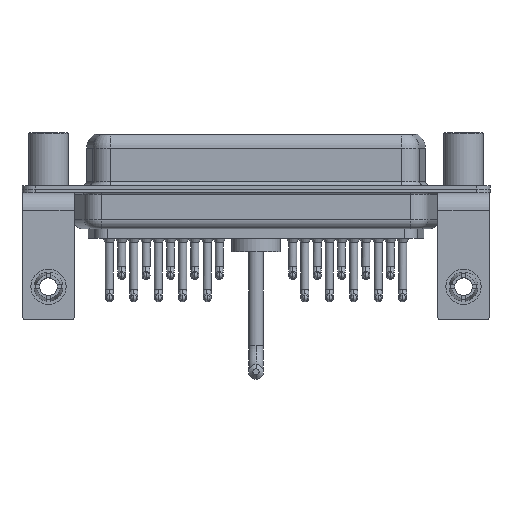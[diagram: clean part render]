
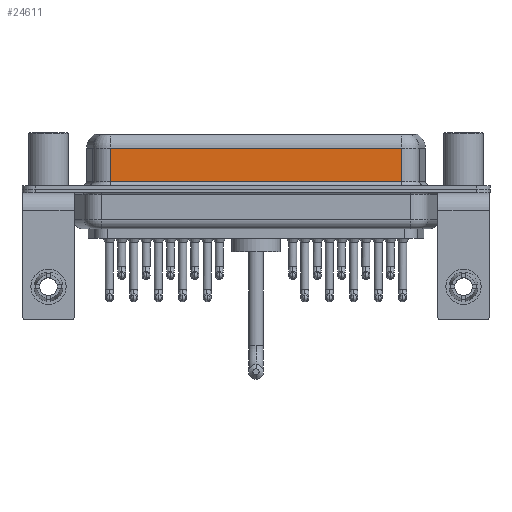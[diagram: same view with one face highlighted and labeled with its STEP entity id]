
A CAD part, front view. The second image highlights one B-rep face of the part: STEP entity #24611.
In plain terms, the highlighted planar face has unit normal (0, -1, 0).
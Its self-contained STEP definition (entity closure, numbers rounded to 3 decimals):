
#1301 = DIRECTION ( 'NONE',  ( 0., 0., 1. ) ) ;
#2319 = DIRECTION ( 'NONE',  ( 1., 0., 0. ) ) ;
#3087 = ORIENTED_EDGE ( 'NONE', *, *, #19730, .T. ) ;
#3514 = EDGE_CURVE ( 'NONE', #24640, #5284, #23763, .T. ) ;
#4156 = CARTESIAN_POINT ( 'NONE',  ( 40.037, -3.95, 4.65 ) ) ;
#4439 = ORIENTED_EDGE ( 'NONE', *, *, #3514, .T. ) ;
#4939 = LINE ( 'NONE', #9287, #15306 ) ;
#5242 = CARTESIAN_POINT ( 'NONE',  ( 7.013, -3.95, 4.65 ) ) ;
#5284 = VERTEX_POINT ( 'NONE', #23367 ) ;
#5513 = FACE_OUTER_BOUND ( 'NONE', #15312, .T. ) ;
#6496 = LINE ( 'NONE', #8418, #7118 ) ;
#7118 = VECTOR ( 'NONE', #2319, 1000. ) ;
#7659 = DIRECTION ( 'NONE',  ( 0., 0., -1. ) ) ;
#8418 = CARTESIAN_POINT ( 'NONE',  ( 40.037, -3.95, 0.9 ) ) ;
#9287 = CARTESIAN_POINT ( 'NONE',  ( 40.037, -3.95, 4.65 ) ) ;
#9983 = DIRECTION ( 'NONE',  ( 0., 1., 0. ) ) ;
#10542 = ORIENTED_EDGE ( 'NONE', *, *, #12055, .F. ) ;
#10940 = VECTOR ( 'NONE', #7659, 1000. ) ;
#11571 = DIRECTION ( 'NONE',  ( -1., 0., 0. ) ) ;
#11830 = ORIENTED_EDGE ( 'NONE', *, *, #15542, .T. ) ;
#11839 = DIRECTION ( 'NONE',  ( 0., 0., -1. ) ) ;
#12055 = EDGE_CURVE ( 'NONE', #26077, #12070, #15888, .T. ) ;
#12070 = VERTEX_POINT ( 'NONE', #17413 ) ;
#13465 = CARTESIAN_POINT ( 'NONE',  ( 7.013, -3.95, 6.4 ) ) ;
#13768 = PLANE ( 'NONE',  #24280 ) ;
#15306 = VECTOR ( 'NONE', #11571, 1000. ) ;
#15312 = EDGE_LOOP ( 'NONE', ( #10542, #3087, #4439, #11830 ) ) ;
#15542 = EDGE_CURVE ( 'NONE', #5284, #12070, #6496, .T. ) ;
#15888 = LINE ( 'NONE', #24291, #25602 ) ;
#17413 = CARTESIAN_POINT ( 'NONE',  ( 40.037, -3.95, 0.9 ) ) ;
#19730 = EDGE_CURVE ( 'NONE', #26077, #24640, #4939, .T. ) ;
#23367 = CARTESIAN_POINT ( 'NONE',  ( 7.013, -3.95, 0.9 ) ) ;
#23763 = LINE ( 'NONE', #13465, #10940 ) ;
#23943 = CARTESIAN_POINT ( 'NONE',  ( 40.037, -3.95, 6.4 ) ) ;
#24280 = AXIS2_PLACEMENT_3D ( 'NONE', #23943, #9983, #1301 ) ;
#24291 = CARTESIAN_POINT ( 'NONE',  ( 40.037, -3.95, 6.4 ) ) ;
#24611 = ADVANCED_FACE ( 'NONE', ( #5513 ), #13768, .F. ) ;
#24640 = VERTEX_POINT ( 'NONE', #5242 ) ;
#25602 = VECTOR ( 'NONE', #11839, 1000. ) ;
#26077 = VERTEX_POINT ( 'NONE', #4156 ) ;
